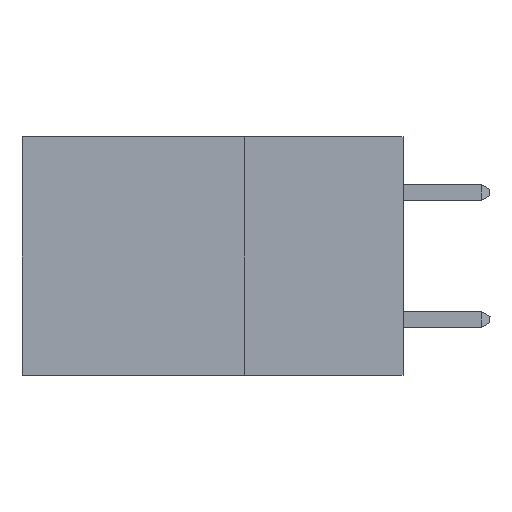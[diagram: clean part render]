
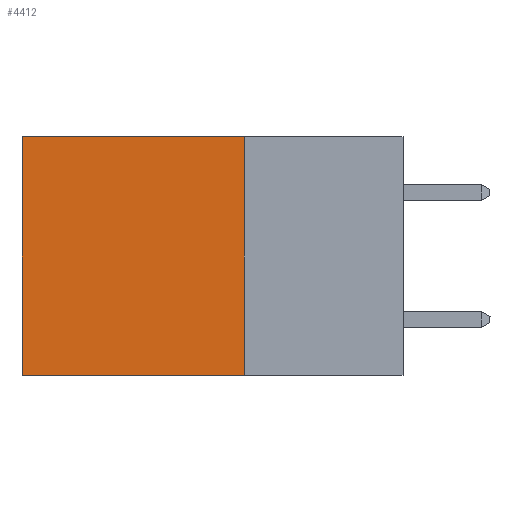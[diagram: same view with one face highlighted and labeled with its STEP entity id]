
A CAD part, left-side view. The second image highlights one B-rep face of the part: STEP entity #4412.
In plain terms, the highlighted planar face has unit normal (-1, 0, 0).
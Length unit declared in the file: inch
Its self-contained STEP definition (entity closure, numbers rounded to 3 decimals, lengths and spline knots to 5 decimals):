
#213 = CARTESIAN_POINT ( 'NONE',  ( 0.2875, 0.25, -0.375 ) ) ;
#314 = ORIENTED_EDGE ( 'NONE', *, *, #3867, .T. ) ;
#345 = DIRECTION ( 'NONE',  ( 0., 0., -1. ) ) ;
#550 = VECTOR ( 'NONE', #1031, 39.37008 ) ;
#1031 = DIRECTION ( 'NONE',  ( 0., 0., -1. ) ) ;
#1521 = CARTESIAN_POINT ( 'NONE',  ( 0.2875, 0.6, -0.375 ) ) ;
#2909 = DIRECTION ( 'NONE',  ( 0., 0., -1. ) ) ;
#3018 = ORIENTED_EDGE ( 'NONE', *, *, #15114, .F. ) ;
#3470 = VECTOR ( 'NONE', #2909, 39.37008 ) ;
#3867 = EDGE_CURVE ( 'NONE', #16335, #11966, #10987, .T. ) ;
#4412 = ADVANCED_FACE ( 'NONE', ( #14374 ), #16313, .F. ) ;
#4719 = CARTESIAN_POINT ( 'NONE',  ( 0.2875, 0.6, 0. ) ) ;
#5388 = CARTESIAN_POINT ( 'NONE',  ( 0.2875, 0.25, 0. ) ) ;
#6187 = DIRECTION ( 'NONE',  ( 1., 0., 0. ) ) ;
#6413 = LINE ( 'NONE', #18249, #18260 ) ;
#7358 = LINE ( 'NONE', #10909, #550 ) ;
#8176 = ORIENTED_EDGE ( 'NONE', *, *, #10269, .T. ) ;
#8830 = VERTEX_POINT ( 'NONE', #17039 ) ;
#10269 = EDGE_CURVE ( 'NONE', #8830, #16335, #17773, .T. ) ;
#10909 = CARTESIAN_POINT ( 'NONE',  ( 0.2875, 0.25, -0.375 ) ) ;
#10987 = LINE ( 'NONE', #1521, #3470 ) ;
#11219 = DIRECTION ( 'NONE',  ( 0., 1., 0. ) ) ;
#11966 = VERTEX_POINT ( 'NONE', #17847 ) ;
#12434 = AXIS2_PLACEMENT_3D ( 'NONE', #213, #6187, #345 ) ;
#12679 = EDGE_LOOP ( 'NONE', ( #314, #3018, #16267, #8176 ) ) ;
#12969 = VECTOR ( 'NONE', #11219, 39.37008 ) ;
#13767 = CARTESIAN_POINT ( 'NONE',  ( 0.2875, 0.25, -0.375 ) ) ;
#13986 = VERTEX_POINT ( 'NONE', #13767 ) ;
#14237 = EDGE_CURVE ( 'NONE', #8830, #13986, #7358, .T. ) ;
#14374 = FACE_OUTER_BOUND ( 'NONE', #12679, .T. ) ;
#15114 = EDGE_CURVE ( 'NONE', #13986, #11966, #6413, .T. ) ;
#16267 = ORIENTED_EDGE ( 'NONE', *, *, #14237, .F. ) ;
#16313 = PLANE ( 'NONE',  #12434 ) ;
#16335 = VERTEX_POINT ( 'NONE', #4719 ) ;
#16693 = DIRECTION ( 'NONE',  ( 0., 1., 0. ) ) ;
#17039 = CARTESIAN_POINT ( 'NONE',  ( 0.2875, 0.25, 0. ) ) ;
#17773 = LINE ( 'NONE', #5388, #12969 ) ;
#17847 = CARTESIAN_POINT ( 'NONE',  ( 0.2875, 0.6, -0.375 ) ) ;
#18249 = CARTESIAN_POINT ( 'NONE',  ( 0.2875, 0.25, -0.375 ) ) ;
#18260 = VECTOR ( 'NONE', #16693, 39.37008 ) ;
